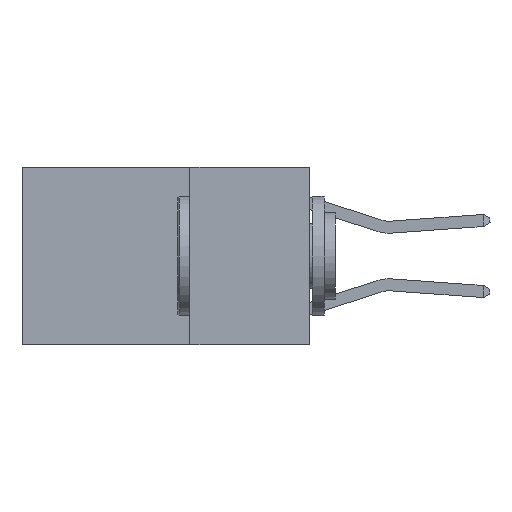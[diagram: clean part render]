
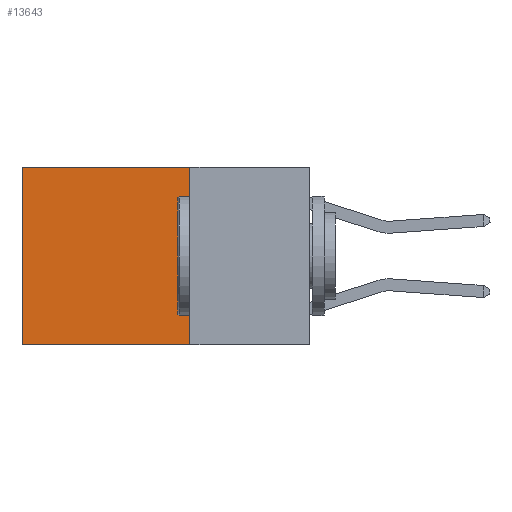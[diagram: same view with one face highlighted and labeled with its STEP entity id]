
A CAD part, left-side view. The second image highlights one B-rep face of the part: STEP entity #13643.
In plain terms, the highlighted planar face has unit normal (-1, 0, 0).
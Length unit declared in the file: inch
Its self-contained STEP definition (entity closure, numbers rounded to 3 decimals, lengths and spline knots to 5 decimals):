
#878 = EDGE_CURVE ( 'NONE', #6073, #7058, #18711, .T. ) ;
#1708 = VECTOR ( 'NONE', #3836, 39.37008 ) ;
#1820 = DIRECTION ( 'NONE',  ( 0., 1., 0. ) ) ;
#3836 = DIRECTION ( 'NONE',  ( 0., 0., -1. ) ) ;
#4251 = ORIENTED_EDGE ( 'NONE', *, *, #878, .F. ) ;
#4326 = ORIENTED_EDGE ( 'NONE', *, *, #12118, .T. ) ;
#5194 = CARTESIAN_POINT ( 'NONE',  ( 0.2625, 0.25, -0.37 ) ) ;
#6073 = VERTEX_POINT ( 'NONE', #5194 ) ;
#6712 = DIRECTION ( 'NONE',  ( 0., 0., -1. ) ) ;
#7058 = VERTEX_POINT ( 'NONE', #19877 ) ;
#8241 = DIRECTION ( 'NONE',  ( 0., 0., -1. ) ) ;
#9466 = CARTESIAN_POINT ( 'NONE',  ( 0.2625, 0.25, 0. ) ) ;
#11464 = ORIENTED_EDGE ( 'NONE', *, *, #28965, .F. ) ;
#12118 = EDGE_CURVE ( 'NONE', #15260, #24802, #18620, .T. ) ;
#13643 = ADVANCED_FACE ( 'NONE', ( #26739 ), #20024, .F. ) ;
#14928 = CARTESIAN_POINT ( 'NONE',  ( 0.2625, 0.25, 0. ) ) ;
#15260 = VERTEX_POINT ( 'NONE', #9466 ) ;
#15387 = DIRECTION ( 'NONE',  ( 1., 0., 0. ) ) ;
#15885 = EDGE_LOOP ( 'NONE', ( #30423, #4251, #11464, #4326 ) ) ;
#16491 = CARTESIAN_POINT ( 'NONE',  ( 0.2625, 0.6, 0. ) ) ;
#16769 = EDGE_CURVE ( 'NONE', #24802, #7058, #28017, .T. ) ;
#17089 = VECTOR ( 'NONE', #1820, 39.37008 ) ;
#17810 = CARTESIAN_POINT ( 'NONE',  ( 0.2625, 0.25, 0. ) ) ;
#18620 = LINE ( 'NONE', #23310, #28754 ) ;
#18711 = LINE ( 'NONE', #18862, #17089 ) ;
#18862 = CARTESIAN_POINT ( 'NONE',  ( 0.2625, 0.25, -0.37 ) ) ;
#18878 = AXIS2_PLACEMENT_3D ( 'NONE', #14928, #15387, #8241 ) ;
#19877 = CARTESIAN_POINT ( 'NONE',  ( 0.2625, 0.6, -0.37 ) ) ;
#20024 = PLANE ( 'NONE',  #18878 ) ;
#22241 = CARTESIAN_POINT ( 'NONE',  ( 0.2625, 0.6, 0. ) ) ;
#22650 = LINE ( 'NONE', #17810, #1708 ) ;
#23310 = CARTESIAN_POINT ( 'NONE',  ( 0.2625, 0.25, 0. ) ) ;
#24802 = VERTEX_POINT ( 'NONE', #22241 ) ;
#26739 = FACE_OUTER_BOUND ( 'NONE', #15885, .T. ) ;
#28017 = LINE ( 'NONE', #16491, #29376 ) ;
#28123 = DIRECTION ( 'NONE',  ( 0., 1., 0. ) ) ;
#28754 = VECTOR ( 'NONE', #28123, 39.37008 ) ;
#28965 = EDGE_CURVE ( 'NONE', #15260, #6073, #22650, .T. ) ;
#29376 = VECTOR ( 'NONE', #6712, 39.37008 ) ;
#30423 = ORIENTED_EDGE ( 'NONE', *, *, #16769, .T. ) ;
